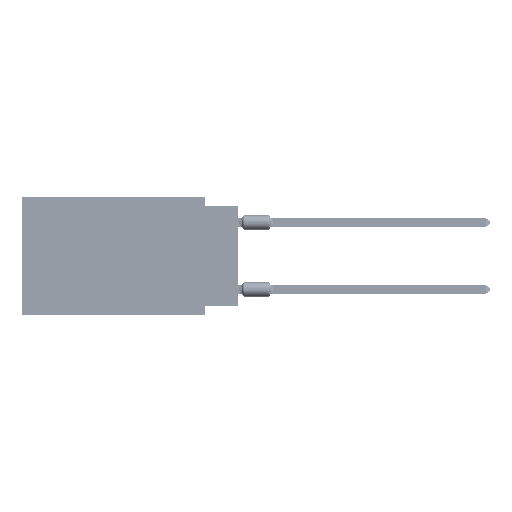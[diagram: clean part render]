
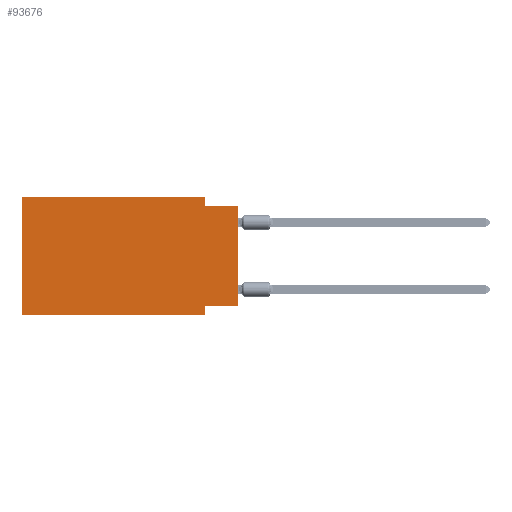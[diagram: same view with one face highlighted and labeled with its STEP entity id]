
A CAD part, left-side view. The second image highlights one B-rep face of the part: STEP entity #93676.
In plain terms, the highlighted planar face has unit normal (-1, 0, 0).
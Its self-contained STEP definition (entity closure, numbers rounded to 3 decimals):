
#2283 = DIRECTION ( 'NONE',  ( 0., -1., 0. ) ) ;
#3046 = EDGE_CURVE ( 'NONE', #5972, #57781, #54595, .T. ) ;
#4671 = VERTEX_POINT ( 'NONE', #12266 ) ;
#5972 = VERTEX_POINT ( 'NONE', #12873 ) ;
#6467 = AXIS2_PLACEMENT_3D ( 'NONE', #74890, #89594, #30236 ) ;
#9324 = PLANE ( 'NONE',  #6467 ) ;
#9496 = CARTESIAN_POINT ( 'NONE',  ( 0., 2.54, -8.89 ) ) ;
#10347 = LINE ( 'NONE', #23213, #11457 ) ;
#11457 = VECTOR ( 'NONE', #38891, 1000. ) ;
#12266 = CARTESIAN_POINT ( 'NONE',  ( 0., 16.383, 0. ) ) ;
#12873 = CARTESIAN_POINT ( 'NONE',  ( 0., 0., -8.255 ) ) ;
#13229 = EDGE_CURVE ( 'NONE', #29308, #62894, #51010, .T. ) ;
#16036 = VECTOR ( 'NONE', #76339, 1000. ) ;
#16293 = ORIENTED_EDGE ( 'NONE', *, *, #88893, .F. ) ;
#20274 = LINE ( 'NONE', #42608, #67778 ) ;
#23213 = CARTESIAN_POINT ( 'NONE',  ( 0., 0., -8.255 ) ) ;
#25146 = CARTESIAN_POINT ( 'NONE',  ( 0., 0., 0. ) ) ;
#27666 = ORIENTED_EDGE ( 'NONE', *, *, #87694, .T. ) ;
#29308 = VERTEX_POINT ( 'NONE', #79836 ) ;
#30236 = DIRECTION ( 'NONE',  ( 0., 0., -1. ) ) ;
#32246 = ORIENTED_EDGE ( 'NONE', *, *, #53673, .F. ) ;
#37556 = VECTOR ( 'NONE', #40359, 1000. ) ;
#38891 = DIRECTION ( 'NONE',  ( 0., 1., 0. ) ) ;
#40359 = DIRECTION ( 'NONE',  ( 0., 0., 1. ) ) ;
#41850 = ORIENTED_EDGE ( 'NONE', *, *, #13229, .F. ) ;
#42392 = VECTOR ( 'NONE', #78668, 1000. ) ;
#42608 = CARTESIAN_POINT ( 'NONE',  ( 0., 16.383, 0. ) ) ;
#43434 = CARTESIAN_POINT ( 'NONE',  ( 0., 2.54, -8.89 ) ) ;
#44068 = EDGE_CURVE ( 'NONE', #67883, #65915, #59275, .T. ) ;
#44840 = DIRECTION ( 'NONE',  ( 0., 0., -1. ) ) ;
#45063 = ORIENTED_EDGE ( 'NONE', *, *, #54977, .F. ) ;
#46529 = CARTESIAN_POINT ( 'NONE',  ( 0., 16.383, -8.89 ) ) ;
#46917 = VECTOR ( 'NONE', #72146, 1000. ) ;
#47828 = CARTESIAN_POINT ( 'NONE',  ( 0., 0., -0.635 ) ) ;
#49255 = DIRECTION ( 'NONE',  ( 0., 0., 1. ) ) ;
#51010 = LINE ( 'NONE', #43434, #75941 ) ;
#51615 = ORIENTED_EDGE ( 'NONE', *, *, #44068, .F. ) ;
#51883 = VERTEX_POINT ( 'NONE', #46529 ) ;
#53673 = EDGE_CURVE ( 'NONE', #65915, #57781, #90586, .T. ) ;
#54595 = LINE ( 'NONE', #25146, #37556 ) ;
#54794 = ORIENTED_EDGE ( 'NONE', *, *, #74797, .F. ) ;
#54977 = EDGE_CURVE ( 'NONE', #51883, #4671, #20274, .T. ) ;
#57759 = CARTESIAN_POINT ( 'NONE',  ( 0., 16.383, 0. ) ) ;
#57781 = VERTEX_POINT ( 'NONE', #89491 ) ;
#58238 = LINE ( 'NONE', #57759, #42392 ) ;
#59275 = LINE ( 'NONE', #79243, #46917 ) ;
#62894 = VERTEX_POINT ( 'NONE', #9496 ) ;
#65915 = VERTEX_POINT ( 'NONE', #77140 ) ;
#66416 = CARTESIAN_POINT ( 'NONE',  ( 0., 16.383, -8.89 ) ) ;
#67357 = LINE ( 'NONE', #66416, #79599 ) ;
#67778 = VECTOR ( 'NONE', #49255, 1000. ) ;
#67883 = VERTEX_POINT ( 'NONE', #84000 ) ;
#72146 = DIRECTION ( 'NONE',  ( 0., 0., -1. ) ) ;
#74412 = FACE_OUTER_BOUND ( 'NONE', #88886, .T. ) ;
#74797 = EDGE_CURVE ( 'NONE', #4671, #67883, #58238, .T. ) ;
#74890 = CARTESIAN_POINT ( 'NONE',  ( 0., 16.383, 0. ) ) ;
#75941 = VECTOR ( 'NONE', #44840, 1000. ) ;
#76339 = DIRECTION ( 'NONE',  ( 0., -1., 0. ) ) ;
#77140 = CARTESIAN_POINT ( 'NONE',  ( 0., 2.54, -0.635 ) ) ;
#77665 = ORIENTED_EDGE ( 'NONE', *, *, #3046, .T. ) ;
#78668 = DIRECTION ( 'NONE',  ( 0., -1., 0. ) ) ;
#79243 = CARTESIAN_POINT ( 'NONE',  ( 0., 2.54, 0. ) ) ;
#79599 = VECTOR ( 'NONE', #2283, 1000. ) ;
#79836 = CARTESIAN_POINT ( 'NONE',  ( 0., 2.54, -8.255 ) ) ;
#84000 = CARTESIAN_POINT ( 'NONE',  ( 0., 2.54, 0. ) ) ;
#87694 = EDGE_CURVE ( 'NONE', #51883, #62894, #67357, .T. ) ;
#88886 = EDGE_LOOP ( 'NONE', ( #77665, #32246, #51615, #54794, #45063, #27666, #41850, #16293 ) ) ;
#88893 = EDGE_CURVE ( 'NONE', #5972, #29308, #10347, .T. ) ;
#89491 = CARTESIAN_POINT ( 'NONE',  ( 0., 0., -0.635 ) ) ;
#89594 = DIRECTION ( 'NONE',  ( 1., 0., 0. ) ) ;
#90586 = LINE ( 'NONE', #47828, #16036 ) ;
#93676 = ADVANCED_FACE ( 'NONE', ( #74412 ), #9324, .F. ) ;
